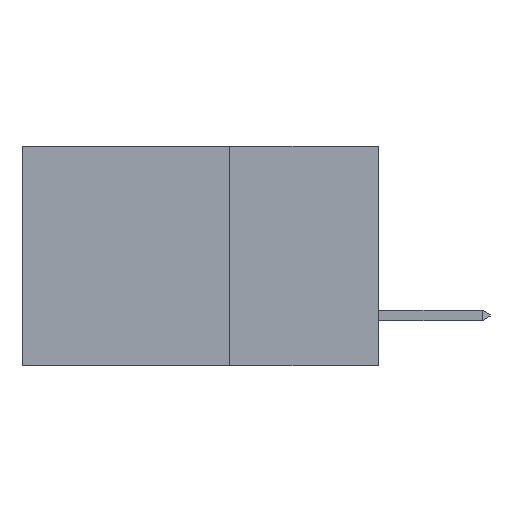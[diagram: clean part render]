
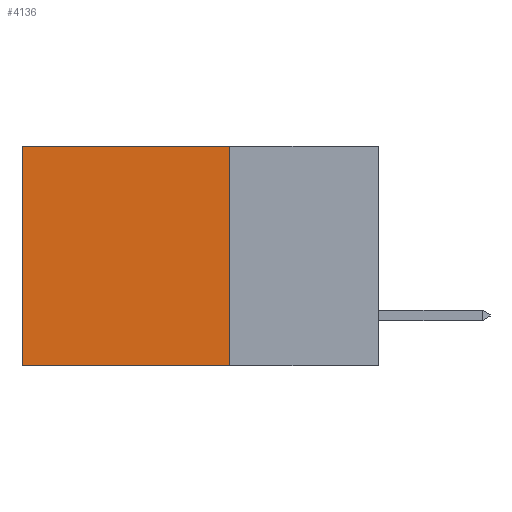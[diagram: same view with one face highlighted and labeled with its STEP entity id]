
A CAD part, left-side view. The second image highlights one B-rep face of the part: STEP entity #4136.
In plain terms, the highlighted planar face has unit normal (-1, 0, 0).
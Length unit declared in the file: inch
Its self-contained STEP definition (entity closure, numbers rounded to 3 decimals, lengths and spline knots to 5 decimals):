
#259 = VERTEX_POINT ( 'NONE', #10911 ) ;
#577 = CARTESIAN_POINT ( 'NONE',  ( 0.298, 0.25, -0.37 ) ) ;
#1491 = DIRECTION ( 'NONE',  ( 0., 1., 0. ) ) ;
#1576 = CARTESIAN_POINT ( 'NONE',  ( 0.298, 0.25, 0. ) ) ;
#2657 = CARTESIAN_POINT ( 'NONE',  ( 0.298, 0.6, 0. ) ) ;
#3193 = EDGE_CURVE ( 'NONE', #11397, #4610, #13826, .T. ) ;
#3779 = PLANE ( 'NONE',  #4894 ) ;
#4136 = ADVANCED_FACE ( 'NONE', ( #5034 ), #3779, .F. ) ;
#4277 = VECTOR ( 'NONE', #1491, 39.37008 ) ;
#4610 = VERTEX_POINT ( 'NONE', #14053 ) ;
#4894 = AXIS2_PLACEMENT_3D ( 'NONE', #7654, #7639, #6751 ) ;
#5034 = FACE_OUTER_BOUND ( 'NONE', #12228, .T. ) ;
#5124 = VECTOR ( 'NONE', #12688, 39.37008 ) ;
#5275 = EDGE_CURVE ( 'NONE', #14461, #4610, #7911, .T. ) ;
#6751 = DIRECTION ( 'NONE',  ( 0., 0., -1. ) ) ;
#7552 = VECTOR ( 'NONE', #14273, 39.37008 ) ;
#7639 = DIRECTION ( 'NONE',  ( 1., 0., 0. ) ) ;
#7654 = CARTESIAN_POINT ( 'NONE',  ( 0.298, 0.25, 0. ) ) ;
#7911 = LINE ( 'NONE', #12670, #7552 ) ;
#9988 = ORIENTED_EDGE ( 'NONE', *, *, #5275, .T. ) ;
#10750 = ORIENTED_EDGE ( 'NONE', *, *, #11024, .T. ) ;
#10911 = CARTESIAN_POINT ( 'NONE',  ( 0.298, 0.25, 0. ) ) ;
#11024 = EDGE_CURVE ( 'NONE', #259, #14461, #15084, .T. ) ;
#11397 = VERTEX_POINT ( 'NONE', #11946 ) ;
#11399 = ORIENTED_EDGE ( 'NONE', *, *, #3193, .F. ) ;
#11518 = CARTESIAN_POINT ( 'NONE',  ( 0.298, 0.25, 0. ) ) ;
#11946 = CARTESIAN_POINT ( 'NONE',  ( 0.298, 0.25, -0.37 ) ) ;
#12228 = EDGE_LOOP ( 'NONE', ( #9988, #11399, #13697, #10750 ) ) ;
#12670 = CARTESIAN_POINT ( 'NONE',  ( 0.298, 0.6, 0. ) ) ;
#12688 = DIRECTION ( 'NONE',  ( 0., 0., -1. ) ) ;
#13545 = DIRECTION ( 'NONE',  ( 0., 1., 0. ) ) ;
#13697 = ORIENTED_EDGE ( 'NONE', *, *, #15223, .F. ) ;
#13826 = LINE ( 'NONE', #577, #4277 ) ;
#14053 = CARTESIAN_POINT ( 'NONE',  ( 0.298, 0.6, -0.37 ) ) ;
#14249 = LINE ( 'NONE', #11518, #5124 ) ;
#14273 = DIRECTION ( 'NONE',  ( 0., 0., -1. ) ) ;
#14461 = VERTEX_POINT ( 'NONE', #2657 ) ;
#14733 = VECTOR ( 'NONE', #13545, 39.37008 ) ;
#15084 = LINE ( 'NONE', #1576, #14733 ) ;
#15223 = EDGE_CURVE ( 'NONE', #259, #11397, #14249, .T. ) ;
